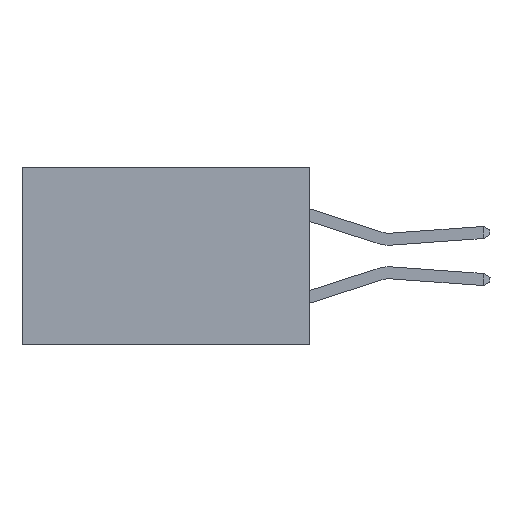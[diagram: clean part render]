
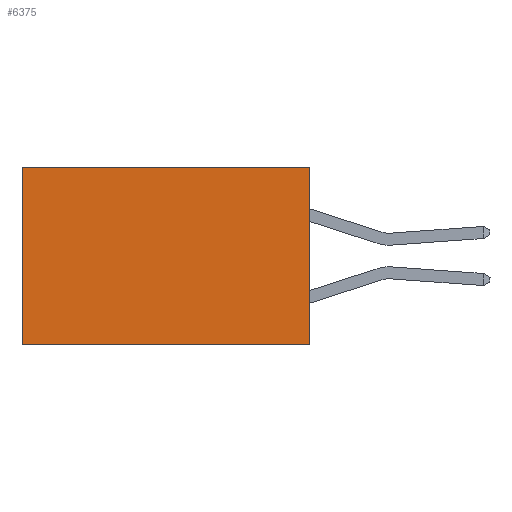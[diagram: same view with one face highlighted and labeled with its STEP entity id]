
A CAD part, left-side view. The second image highlights one B-rep face of the part: STEP entity #6375.
In plain terms, the highlighted planar face has unit normal (-1, 0, 0).
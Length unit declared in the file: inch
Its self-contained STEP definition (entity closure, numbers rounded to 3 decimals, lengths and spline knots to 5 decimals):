
#411 = CARTESIAN_POINT ( 'NONE',  ( 0.2615, 0., -0.37 ) ) ;
#889 = ORIENTED_EDGE ( 'NONE', *, *, #13346, .F. ) ;
#1254 = DIRECTION ( 'NONE',  ( 0., 0., -1. ) ) ;
#1304 = DIRECTION ( 'NONE',  ( 1., 0., 0. ) ) ;
#1371 = CARTESIAN_POINT ( 'NONE',  ( 0.2615, 0., -0.37 ) ) ;
#1440 = PLANE ( 'NONE',  #6498 ) ;
#1501 = EDGE_CURVE ( 'NONE', #16796, #20813, #4857, .T. ) ;
#2138 = DIRECTION ( 'NONE',  ( 0., 1., 0. ) ) ;
#2164 = LINE ( 'NONE', #15311, #2681 ) ;
#2681 = VECTOR ( 'NONE', #6883, 39.37008 ) ;
#3458 = CARTESIAN_POINT ( 'NONE',  ( 0.2615, 0.6, -0.37 ) ) ;
#4857 = LINE ( 'NONE', #7203, #5379 ) ;
#4884 = VECTOR ( 'NONE', #18938, 39.37008 ) ;
#5379 = VECTOR ( 'NONE', #2138, 39.37008 ) ;
#6375 = ADVANCED_FACE ( 'NONE', ( #19181 ), #1440, .F. ) ;
#6498 = AXIS2_PLACEMENT_3D ( 'NONE', #1371, #1304, #1254 ) ;
#6883 = DIRECTION ( 'NONE',  ( 0., 1., 0. ) ) ;
#7155 = ORIENTED_EDGE ( 'NONE', *, *, #20945, .T. ) ;
#7173 = EDGE_LOOP ( 'NONE', ( #7155, #17481, #889, #20913 ) ) ;
#7203 = CARTESIAN_POINT ( 'NONE',  ( 0.2615, 0., -0.37 ) ) ;
#7373 = VECTOR ( 'NONE', #10966, 39.37008 ) ;
#7549 = CARTESIAN_POINT ( 'NONE',  ( 0.2615, 0., -0.37 ) ) ;
#8805 = CARTESIAN_POINT ( 'NONE',  ( 0.2615, 0.6, -0.37 ) ) ;
#9364 = LINE ( 'NONE', #8805, #4884 ) ;
#9812 = CARTESIAN_POINT ( 'NONE',  ( 0.2615, 0.6, 0. ) ) ;
#10966 = DIRECTION ( 'NONE',  ( 0., 0., -1. ) ) ;
#11907 = LINE ( 'NONE', #7549, #7373 ) ;
#13186 = EDGE_CURVE ( 'NONE', #19262, #18952, #2164, .T. ) ;
#13346 = EDGE_CURVE ( 'NONE', #19262, #16796, #11907, .T. ) ;
#15311 = CARTESIAN_POINT ( 'NONE',  ( 0.2615, 0., 0. ) ) ;
#16796 = VERTEX_POINT ( 'NONE', #411 ) ;
#17481 = ORIENTED_EDGE ( 'NONE', *, *, #1501, .F. ) ;
#18938 = DIRECTION ( 'NONE',  ( 0., 0., -1. ) ) ;
#18952 = VERTEX_POINT ( 'NONE', #9812 ) ;
#19046 = CARTESIAN_POINT ( 'NONE',  ( 0.2615, 0., 0. ) ) ;
#19181 = FACE_OUTER_BOUND ( 'NONE', #7173, .T. ) ;
#19262 = VERTEX_POINT ( 'NONE', #19046 ) ;
#20813 = VERTEX_POINT ( 'NONE', #3458 ) ;
#20913 = ORIENTED_EDGE ( 'NONE', *, *, #13186, .T. ) ;
#20945 = EDGE_CURVE ( 'NONE', #18952, #20813, #9364, .T. ) ;
